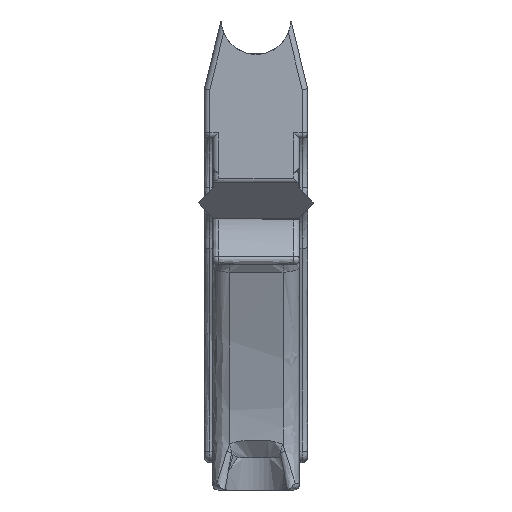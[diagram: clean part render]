
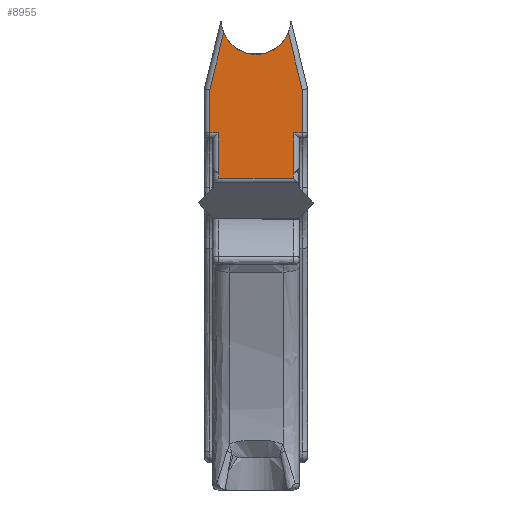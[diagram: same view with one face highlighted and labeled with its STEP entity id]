
A CAD part, front view. The second image highlights one B-rep face of the part: STEP entity #8955.
In plain terms, the highlighted planar face has unit normal (0, -1, 0).
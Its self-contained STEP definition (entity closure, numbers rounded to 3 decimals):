
#946=FACE_OUTER_BOUND('',#1444,.T.);
#1444=EDGE_LOOP('',(#8056,#8057,#8058,#8059,#8060,#8061,#8062,#8063,#8064,
#8065,#8066,#8067,#8068,#8069));
#1659=CIRCLE('',#9561,6.4);
#2465=LINE('',#18951,#3333);
#2476=LINE('',#18978,#3344);
#2486=LINE('',#18995,#3354);
#2498=LINE('',#19024,#3366);
#2499=LINE('',#19027,#3367);
#2500=LINE('',#19029,#3368);
#2501=LINE('',#19031,#3369);
#2502=LINE('',#19033,#3370);
#2503=LINE('',#19037,#3371);
#2504=LINE('',#19039,#3372);
#2505=LINE('',#19040,#3373);
#2506=LINE('',#19042,#3374);
#2507=LINE('',#19043,#3375);
#3333=VECTOR('',#11471,10.);
#3344=VECTOR('',#11498,10.);
#3354=VECTOR('',#11514,10.);
#3366=VECTOR('',#11548,10.);
#3367=VECTOR('',#11551,10.);
#3368=VECTOR('',#11552,10.);
#3369=VECTOR('',#11553,10.);
#3370=VECTOR('',#11554,10.);
#3371=VECTOR('',#11557,10.);
#3372=VECTOR('',#11558,10.);
#3373=VECTOR('',#11559,10.);
#3374=VECTOR('',#11560,1.);
#3375=VECTOR('',#11561,10.);
#4200=VERTEX_POINT('',#18947);
#4202=VERTEX_POINT('',#18950);
#4209=VERTEX_POINT('',#18975);
#4210=VERTEX_POINT('',#18977);
#4214=VERTEX_POINT('',#18994);
#4220=VERTEX_POINT('',#19022);
#4221=VERTEX_POINT('',#19026);
#4222=VERTEX_POINT('',#19028);
#4223=VERTEX_POINT('',#19030);
#4224=VERTEX_POINT('',#19032);
#4225=VERTEX_POINT('',#19034);
#4226=VERTEX_POINT('',#19036);
#4227=VERTEX_POINT('',#19038);
#4228=VERTEX_POINT('',#19041);
#5477=EDGE_CURVE('',#4202,#4200,#2465,.T.);
#5491=EDGE_CURVE('',#4210,#4209,#2476,.T.);
#5502=EDGE_CURVE('',#4210,#4214,#2486,.T.);
#5517=EDGE_CURVE('',#4220,#4209,#2498,.T.);
#5518=EDGE_CURVE('',#4221,#4200,#2499,.T.);
#5519=EDGE_CURVE('',#4222,#4221,#2500,.T.);
#5520=EDGE_CURVE('',#4223,#4222,#2501,.T.);
#5521=EDGE_CURVE('',#4224,#4223,#2502,.T.);
#5522=EDGE_CURVE('',#4224,#4225,#1659,.T.);
#5523=EDGE_CURVE('',#4226,#4225,#2503,.T.);
#5524=EDGE_CURVE('',#4227,#4226,#2504,.T.);
#5525=EDGE_CURVE('',#4214,#4227,#2505,.T.);
#5526=EDGE_CURVE('',#4228,#4220,#2506,.T.);
#5527=EDGE_CURVE('',#4202,#4228,#2507,.T.);
#8056=ORIENTED_EDGE('',*,*,#5518,.F.);
#8057=ORIENTED_EDGE('',*,*,#5519,.F.);
#8058=ORIENTED_EDGE('',*,*,#5520,.F.);
#8059=ORIENTED_EDGE('',*,*,#5521,.F.);
#8060=ORIENTED_EDGE('',*,*,#5522,.T.);
#8061=ORIENTED_EDGE('',*,*,#5523,.F.);
#8062=ORIENTED_EDGE('',*,*,#5524,.F.);
#8063=ORIENTED_EDGE('',*,*,#5525,.F.);
#8064=ORIENTED_EDGE('',*,*,#5502,.F.);
#8065=ORIENTED_EDGE('',*,*,#5491,.T.);
#8066=ORIENTED_EDGE('',*,*,#5517,.F.);
#8067=ORIENTED_EDGE('',*,*,#5526,.F.);
#8068=ORIENTED_EDGE('',*,*,#5527,.F.);
#8069=ORIENTED_EDGE('',*,*,#5477,.T.);
#8495=PLANE('',#9560);
#8955=ADVANCED_FACE('',(#946),#8495,.T.);
#9560=AXIS2_PLACEMENT_3D('',#19025,#11549,#11550);
#9561=AXIS2_PLACEMENT_3D('',#19035,#11555,#11556);
#11471=DIRECTION('',(0.707,0.,0.707));
#11498=DIRECTION('',(0.707,0.,-0.707));
#11514=DIRECTION('',(0.,0.,1.));
#11548=DIRECTION('',(0.,0.,1.));
#11549=DIRECTION('center_axis',(0.,-1.,0.));
#11550=DIRECTION('ref_axis',(1.,0.,0.));
#11551=DIRECTION('',(0.,0.,-1.));
#11552=DIRECTION('',(-1.,0.,0.));
#11553=DIRECTION('',(0.,0.,-1.));
#11554=DIRECTION('',(0.234,0.,-0.972));
#11555=DIRECTION('center_axis',(0.,1.,0.));
#11556=DIRECTION('ref_axis',(1.,0.,0.));
#11557=DIRECTION('',(0.234,0.,0.972));
#11558=DIRECTION('',(0.,0.,1.));
#11559=DIRECTION('',(-1.,0.,0.));
#11560=DIRECTION('',(-1.,0.,0.));
#11561=DIRECTION('',(0.,0.,-1.));
#18947=CARTESIAN_POINT('',(14.9,-169.,-12.));
#18950=CARTESIAN_POINT('',(14.786,-169.,-12.114));
#18951=CARTESIAN_POINT('',(15.3,-169.,-11.6));
#18975=CARTESIAN_POINT('',(1.114,-169.,-12.114));
#18977=CARTESIAN_POINT('',(1.,-169.,-12.));
#18978=CARTESIAN_POINT('',(-3.375,-169.,-7.625));
#18994=CARTESIAN_POINT('',(1.,-169.,-4.6));
#18995=CARTESIAN_POINT('',(1.,-169.,-8.575));
#19022=CARTESIAN_POINT('',(1.114,-169.,-12.908));
#19024=CARTESIAN_POINT('',(1.114,-169.,-6.143));
#19025=CARTESIAN_POINT('Origin',(15.9,-169.,2.25));
#19026=CARTESIAN_POINT('',(14.9,-169.,-4.6));
#19027=CARTESIAN_POINT('',(14.9,-169.,4.475));
#19028=CARTESIAN_POINT('',(16.4,-169.,-4.6));
#19029=CARTESIAN_POINT('',(8.675,-169.,-4.6));
#19030=CARTESIAN_POINT('',(16.4,-169.,3.381));
#19031=CARTESIAN_POINT('',(16.4,-169.,-0.213));
#19032=CARTESIAN_POINT('',(13.888,-169.,13.812));
#19033=CARTESIAN_POINT('',(15.054,-169.,8.971));
#19034=CARTESIAN_POINT('',(2.012,-169.,13.812));
#19035=CARTESIAN_POINT('Origin',(7.95,-169.,16.2));
#19036=CARTESIAN_POINT('',(-0.5,-169.,3.381));
#19037=CARTESIAN_POINT('',(-0.193,-169.,4.655));
#19038=CARTESIAN_POINT('',(-0.5,-169.,-4.6));
#19039=CARTESIAN_POINT('',(-0.5,-169.,-0.213));
#19040=CARTESIAN_POINT('',(8.675,-169.,-4.6));
#19041=CARTESIAN_POINT('',(14.786,-169.,-12.908));
#19042=CARTESIAN_POINT('',(15.786,-169.,-12.908));
#19043=CARTESIAN_POINT('',(14.786,-169.,-4.375));
